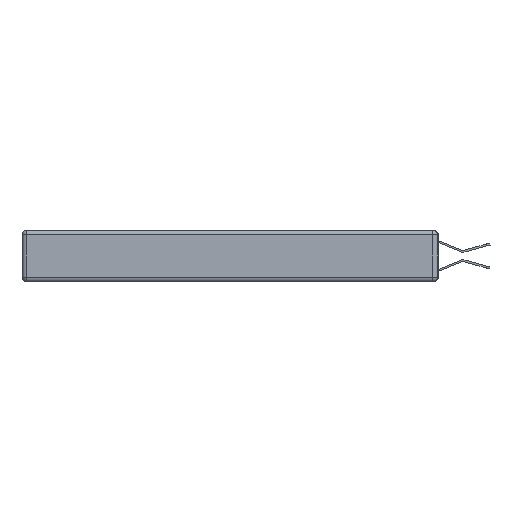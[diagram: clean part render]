
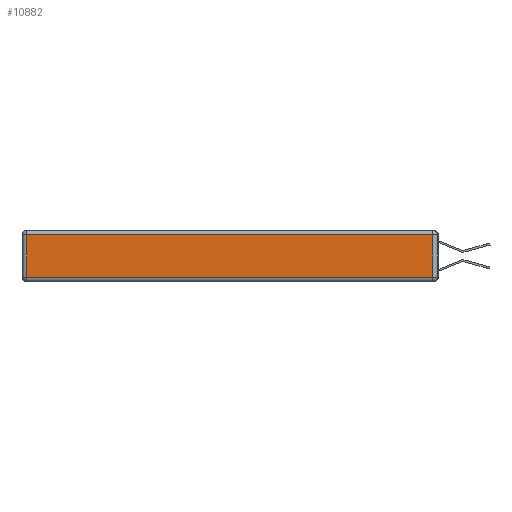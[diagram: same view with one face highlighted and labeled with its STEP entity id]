
A CAD part, left-side view. The second image highlights one B-rep face of the part: STEP entity #10882.
In plain terms, the highlighted planar face has unit normal (-1, 0, 0).
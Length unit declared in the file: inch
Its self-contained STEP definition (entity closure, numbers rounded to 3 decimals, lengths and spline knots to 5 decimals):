
#672 = CARTESIAN_POINT ( 'NONE',  ( 0., 0.03, -0.313 ) ) ;
#747 = CARTESIAN_POINT ( 'NONE',  ( 0., 2.75, -0.03 ) ) ;
#3050 = ORIENTED_EDGE ( 'NONE', *, *, #6172, .T. ) ;
#4531 = CARTESIAN_POINT ( 'NONE',  ( 0., 2.72, -0.03 ) ) ;
#5398 = DIRECTION ( 'NONE',  ( 0., 0., 1. ) ) ;
#5405 = AXIS2_PLACEMENT_3D ( 'NONE', #26388, #26096, #11084 ) ;
#6172 = EDGE_CURVE ( 'NONE', #8088, #24458, #18204, .T. ) ;
#7516 = CARTESIAN_POINT ( 'NONE',  ( 0., 0.03, -0.343 ) ) ;
#8088 = VERTEX_POINT ( 'NONE', #672 ) ;
#8846 = VECTOR ( 'NONE', #21700, 39.37008 ) ;
#9525 = VERTEX_POINT ( 'NONE', #20066 ) ;
#9550 = DIRECTION ( 'NONE',  ( 0., 0., -1. ) ) ;
#10458 = LINE ( 'NONE', #17898, #8846 ) ;
#10882 = ADVANCED_FACE ( 'NONE', ( #22067 ), #21783, .T. ) ;
#11084 = DIRECTION ( 'NONE',  ( 0., 0., 1. ) ) ;
#11105 = CARTESIAN_POINT ( 'NONE',  ( 0., 0.03, -0.03 ) ) ;
#11638 = DIRECTION ( 'NONE',  ( 0., 1., 0. ) ) ;
#12242 = EDGE_CURVE ( 'NONE', #24458, #25275, #13765, .T. ) ;
#13765 = LINE ( 'NONE', #747, #23406 ) ;
#14267 = ORIENTED_EDGE ( 'NONE', *, *, #12242, .T. ) ;
#15493 = ORIENTED_EDGE ( 'NONE', *, *, #20766, .T. ) ;
#15544 = VECTOR ( 'NONE', #9550, 39.37008 ) ;
#15811 = EDGE_LOOP ( 'NONE', ( #15493, #3050, #14267, #22825 ) ) ;
#17898 = CARTESIAN_POINT ( 'NONE',  ( 0., 0., -0.313 ) ) ;
#18204 = LINE ( 'NONE', #7516, #22138 ) ;
#19480 = EDGE_CURVE ( 'NONE', #25275, #9525, #26531, .T. ) ;
#20066 = CARTESIAN_POINT ( 'NONE',  ( 0., 2.72, -0.313 ) ) ;
#20225 = CARTESIAN_POINT ( 'NONE',  ( 0., 2.72, -0.343 ) ) ;
#20766 = EDGE_CURVE ( 'NONE', #9525, #8088, #10458, .T. ) ;
#21700 = DIRECTION ( 'NONE',  ( 0., -1., 0. ) ) ;
#21783 = PLANE ( 'NONE',  #5405 ) ;
#22067 = FACE_OUTER_BOUND ( 'NONE', #15811, .T. ) ;
#22138 = VECTOR ( 'NONE', #5398, 39.37008 ) ;
#22825 = ORIENTED_EDGE ( 'NONE', *, *, #19480, .T. ) ;
#23406 = VECTOR ( 'NONE', #11638, 39.37008 ) ;
#24458 = VERTEX_POINT ( 'NONE', #11105 ) ;
#25275 = VERTEX_POINT ( 'NONE', #4531 ) ;
#26096 = DIRECTION ( 'NONE',  ( -1., 0., 0. ) ) ;
#26388 = CARTESIAN_POINT ( 'NONE',  ( 0., 0., -0.343 ) ) ;
#26531 = LINE ( 'NONE', #20225, #15544 ) ;
